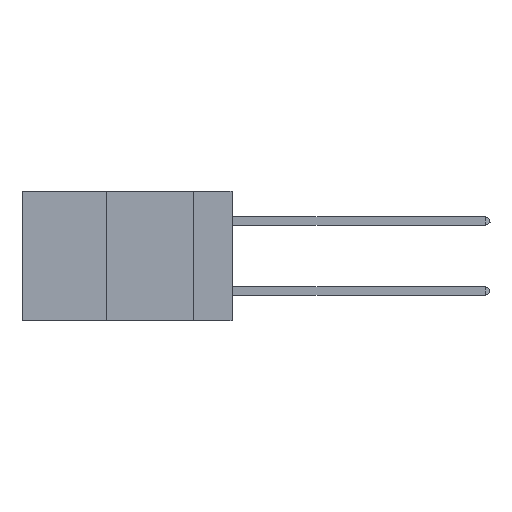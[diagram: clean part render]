
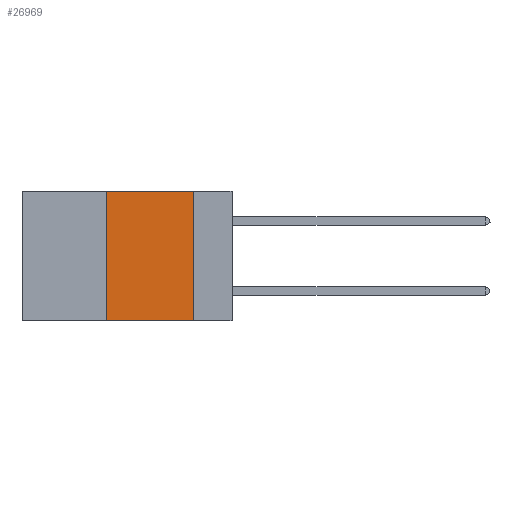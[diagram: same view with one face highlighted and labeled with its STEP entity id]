
A CAD part, left-side view. The second image highlights one B-rep face of the part: STEP entity #26969.
In plain terms, the highlighted planar face has unit normal (-1, 0, 0).
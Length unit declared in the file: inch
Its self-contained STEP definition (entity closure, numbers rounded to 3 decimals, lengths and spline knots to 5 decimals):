
#505 = DIRECTION ( 'NONE',  ( 0., 0., -1. ) ) ;
#1177 = PLANE ( 'NONE',  #10822 ) ;
#2268 = CARTESIAN_POINT ( 'NONE',  ( 0., 0.6, 0. ) ) ;
#2406 = LINE ( 'NONE', #20260, #30941 ) ;
#3203 = EDGE_CURVE ( 'NONE', #30813, #32422, #6955, .T. ) ;
#5013 = DIRECTION ( 'NONE',  ( 0., 0., -1. ) ) ;
#6955 = LINE ( 'NONE', #9699, #30800 ) ;
#7659 = CARTESIAN_POINT ( 'NONE',  ( 0., 0.36, 0. ) ) ;
#7997 = EDGE_CURVE ( 'NONE', #11010, #25991, #13711, .T. ) ;
#9699 = CARTESIAN_POINT ( 'NONE',  ( 0., 0.11, 0. ) ) ;
#10166 = FACE_OUTER_BOUND ( 'NONE', #18532, .T. ) ;
#10822 = AXIS2_PLACEMENT_3D ( 'NONE', #2268, #12919, #5013 ) ;
#11010 = VERTEX_POINT ( 'NONE', #20086 ) ;
#11424 = DIRECTION ( 'NONE',  ( 0., -1., 0. ) ) ;
#12919 = DIRECTION ( 'NONE',  ( 1., 0., 0. ) ) ;
#13711 = LINE ( 'NONE', #7659, #21047 ) ;
#15730 = ORIENTED_EDGE ( 'NONE', *, *, #36074, .F. ) ;
#17599 = CARTESIAN_POINT ( 'NONE',  ( 0., 0.11, -0.37 ) ) ;
#18532 = EDGE_LOOP ( 'NONE', ( #30004, #15730, #21578, #33843 ) ) ;
#20086 = CARTESIAN_POINT ( 'NONE',  ( 0., 0.36, -0.37 ) ) ;
#20260 = CARTESIAN_POINT ( 'NONE',  ( 0., 0.6, -0.37 ) ) ;
#21047 = VECTOR ( 'NONE', #35087, 39.37008 ) ;
#21578 = ORIENTED_EDGE ( 'NONE', *, *, #7997, .F. ) ;
#21860 = CARTESIAN_POINT ( 'NONE',  ( 0., 0.36, 0. ) ) ;
#21898 = VECTOR ( 'NONE', #34456, 39.37008 ) ;
#22521 = CARTESIAN_POINT ( 'NONE',  ( 0., 0.6, 0. ) ) ;
#25991 = VERTEX_POINT ( 'NONE', #21860 ) ;
#26969 = ADVANCED_FACE ( 'NONE', ( #10166 ), #1177, .F. ) ;
#27605 = EDGE_CURVE ( 'NONE', #11010, #32422, #2406, .T. ) ;
#28196 = CARTESIAN_POINT ( 'NONE',  ( 0., 0.11, 0. ) ) ;
#30004 = ORIENTED_EDGE ( 'NONE', *, *, #3203, .F. ) ;
#30800 = VECTOR ( 'NONE', #505, 39.37008 ) ;
#30813 = VERTEX_POINT ( 'NONE', #28196 ) ;
#30941 = VECTOR ( 'NONE', #11424, 39.37008 ) ;
#32422 = VERTEX_POINT ( 'NONE', #17599 ) ;
#33843 = ORIENTED_EDGE ( 'NONE', *, *, #27605, .T. ) ;
#34267 = LINE ( 'NONE', #22521, #21898 ) ;
#34456 = DIRECTION ( 'NONE',  ( 0., -1., 0. ) ) ;
#35087 = DIRECTION ( 'NONE',  ( 0., 0., 1. ) ) ;
#36074 = EDGE_CURVE ( 'NONE', #25991, #30813, #34267, .T. ) ;
